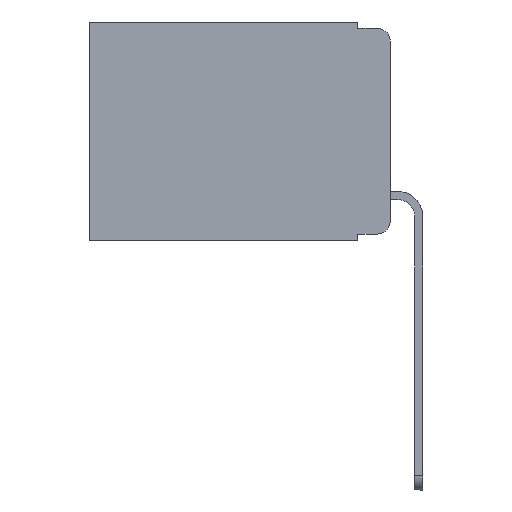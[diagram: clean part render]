
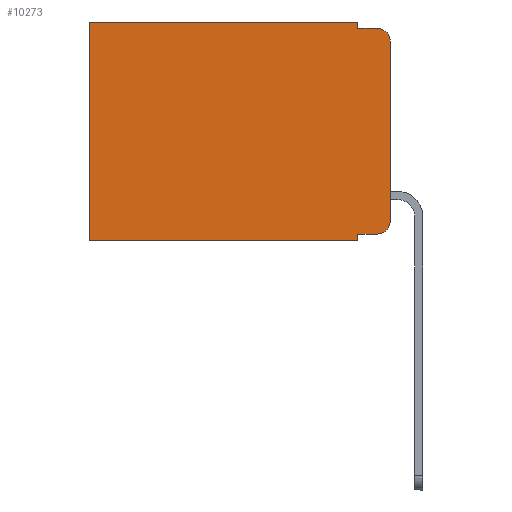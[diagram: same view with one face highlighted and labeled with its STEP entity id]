
A CAD part, left-side view. The second image highlights one B-rep face of the part: STEP entity #10273.
In plain terms, the highlighted planar face has unit normal (-1, 0, 0).
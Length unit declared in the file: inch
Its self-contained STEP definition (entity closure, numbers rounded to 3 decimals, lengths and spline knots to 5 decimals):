
#272 = FACE_OUTER_BOUND ( 'NONE', #5683, .T. ) ;
#402 = CARTESIAN_POINT ( 'NONE',  ( 0.298, 0.051, -0.333 ) ) ;
#705 = VERTEX_POINT ( 'NONE', #9964 ) ;
#1305 = VERTEX_POINT ( 'NONE', #12689 ) ;
#1468 = CIRCLE ( 'NONE', #20230, 0.02 ) ;
#1598 = ORIENTED_EDGE ( 'NONE', *, *, #20343, .F. ) ;
#1930 = PLANE ( 'NONE',  #18754 ) ;
#2007 = CARTESIAN_POINT ( 'NONE',  ( 0.298, 0.02, -0.03 ) ) ;
#2452 = CARTESIAN_POINT ( 'NONE',  ( 0.298, 0.02, -0.01 ) ) ;
#3586 = CARTESIAN_POINT ( 'NONE',  ( 0.298, 0., 0. ) ) ;
#3690 = LINE ( 'NONE', #3586, #3766 ) ;
#3766 = VECTOR ( 'NONE', #14109, 39.37008 ) ;
#3961 = VERTEX_POINT ( 'NONE', #14930 ) ;
#4015 = DIRECTION ( 'NONE',  ( 0., 0., -1. ) ) ;
#4137 = ORIENTED_EDGE ( 'NONE', *, *, #15783, .T. ) ;
#4173 = VECTOR ( 'NONE', #18829, 39.37008 ) ;
#4241 = CARTESIAN_POINT ( 'NONE',  ( 0.298, 0.473, 0. ) ) ;
#4502 = DIRECTION ( 'NONE',  ( -1., 0., 0. ) ) ;
#4708 = CARTESIAN_POINT ( 'NONE',  ( 0.298, 0.051, 0. ) ) ;
#5683 = EDGE_LOOP ( 'NONE', ( #20755, #4137, #12139, #21028, #20273, #18225, #15408, #1598, #11897, #7816 ) ) ;
#6067 = CARTESIAN_POINT ( 'NONE',  ( 0.298, 0., -0.313 ) ) ;
#6158 = VECTOR ( 'NONE', #13902, 39.37008 ) ;
#6461 = EDGE_CURVE ( 'NONE', #9004, #10953, #3690, .T. ) ;
#6889 = VECTOR ( 'NONE', #21784, 39.37008 ) ;
#7030 = DIRECTION ( 'NONE',  ( 1., 0., 0. ) ) ;
#7320 = CARTESIAN_POINT ( 'NONE',  ( 0.298, 0.473, 0. ) ) ;
#7493 = CARTESIAN_POINT ( 'NONE',  ( 0.298, 0.02, -0.313 ) ) ;
#7816 = ORIENTED_EDGE ( 'NONE', *, *, #12599, .T. ) ;
#8092 = LINE ( 'NONE', #9531, #14016 ) ;
#8158 = VERTEX_POINT ( 'NONE', #17077 ) ;
#8767 = DIRECTION ( 'NONE',  ( -1., 0., 0. ) ) ;
#8804 = CARTESIAN_POINT ( 'NONE',  ( 0.298, 0., 0. ) ) ;
#9004 = VERTEX_POINT ( 'NONE', #12047 ) ;
#9333 = VECTOR ( 'NONE', #21646, 39.37008 ) ;
#9531 = CARTESIAN_POINT ( 'NONE',  ( 0.298, 0.051, 0. ) ) ;
#9964 = CARTESIAN_POINT ( 'NONE',  ( 0.298, 0.051, -0.01 ) ) ;
#10273 = ADVANCED_FACE ( 'NONE', ( #272 ), #1930, .F. ) ;
#10521 = CARTESIAN_POINT ( 'NONE',  ( 0.298, 0.051, -0.01 ) ) ;
#10665 = CARTESIAN_POINT ( 'NONE',  ( 0.298, 0.051, -0.333 ) ) ;
#10953 = VERTEX_POINT ( 'NONE', #6067 ) ;
#11064 = VECTOR ( 'NONE', #4015, 39.37008 ) ;
#11520 = VECTOR ( 'NONE', #15269, 39.37008 ) ;
#11543 = LINE ( 'NONE', #13416, #9333 ) ;
#11897 = ORIENTED_EDGE ( 'NONE', *, *, #17903, .T. ) ;
#12047 = CARTESIAN_POINT ( 'NONE',  ( 0.298, 0., -0.03 ) ) ;
#12139 = ORIENTED_EDGE ( 'NONE', *, *, #21716, .F. ) ;
#12599 = EDGE_CURVE ( 'NONE', #8158, #10953, #1468, .T. ) ;
#12689 = CARTESIAN_POINT ( 'NONE',  ( 0.298, 0.051, 0. ) ) ;
#13270 = VERTEX_POINT ( 'NONE', #10665 ) ;
#13335 = LINE ( 'NONE', #4708, #6889 ) ;
#13416 = CARTESIAN_POINT ( 'NONE',  ( 0.298, 0., 0. ) ) ;
#13902 = DIRECTION ( 'NONE',  ( 0., -1., 0. ) ) ;
#14016 = VECTOR ( 'NONE', #14840, 39.37008 ) ;
#14109 = DIRECTION ( 'NONE',  ( 0., 0., -1. ) ) ;
#14168 = EDGE_CURVE ( 'NONE', #17175, #21309, #20979, .T. ) ;
#14840 = DIRECTION ( 'NONE',  ( 0., 0., -1. ) ) ;
#14930 = CARTESIAN_POINT ( 'NONE',  ( 0.298, 0.051, -0.343 ) ) ;
#15119 = CARTESIAN_POINT ( 'NONE',  ( 0.298, 0.473, -0.343 ) ) ;
#15269 = DIRECTION ( 'NONE',  ( 0., 1., 0. ) ) ;
#15350 = LINE ( 'NONE', #402, #6158 ) ;
#15408 = ORIENTED_EDGE ( 'NONE', *, *, #19172, .F. ) ;
#15783 = EDGE_CURVE ( 'NONE', #9004, #18899, #16078, .T. ) ;
#16078 = CIRCLE ( 'NONE', #17141, 0.02 ) ;
#16872 = EDGE_CURVE ( 'NONE', #1305, #17175, #11543, .T. ) ;
#16939 = LINE ( 'NONE', #18820, #11520 ) ;
#17077 = CARTESIAN_POINT ( 'NONE',  ( 0.298, 0.02, -0.333 ) ) ;
#17141 = AXIS2_PLACEMENT_3D ( 'NONE', #2007, #8767, #20730 ) ;
#17175 = VERTEX_POINT ( 'NONE', #7320 ) ;
#17903 = EDGE_CURVE ( 'NONE', #13270, #8158, #15350, .T. ) ;
#17908 = DIRECTION ( 'NONE',  ( 0., 0., -1. ) ) ;
#18174 = EDGE_CURVE ( 'NONE', #1305, #705, #13335, .T. ) ;
#18225 = ORIENTED_EDGE ( 'NONE', *, *, #14168, .T. ) ;
#18754 = AXIS2_PLACEMENT_3D ( 'NONE', #8804, #7030, #18882 ) ;
#18820 = CARTESIAN_POINT ( 'NONE',  ( 0.298, 0., -0.343 ) ) ;
#18829 = DIRECTION ( 'NONE',  ( 0., -1., 0. ) ) ;
#18882 = DIRECTION ( 'NONE',  ( 0., 0., -1. ) ) ;
#18899 = VERTEX_POINT ( 'NONE', #2452 ) ;
#19172 = EDGE_CURVE ( 'NONE', #3961, #21309, #16939, .T. ) ;
#20230 = AXIS2_PLACEMENT_3D ( 'NONE', #7493, #4502, #17908 ) ;
#20273 = ORIENTED_EDGE ( 'NONE', *, *, #16872, .T. ) ;
#20285 = LINE ( 'NONE', #10521, #4173 ) ;
#20343 = EDGE_CURVE ( 'NONE', #13270, #3961, #8092, .T. ) ;
#20730 = DIRECTION ( 'NONE',  ( 0., 0., -1. ) ) ;
#20755 = ORIENTED_EDGE ( 'NONE', *, *, #6461, .F. ) ;
#20979 = LINE ( 'NONE', #4241, #11064 ) ;
#21028 = ORIENTED_EDGE ( 'NONE', *, *, #18174, .F. ) ;
#21309 = VERTEX_POINT ( 'NONE', #15119 ) ;
#21646 = DIRECTION ( 'NONE',  ( 0., 1., 0. ) ) ;
#21716 = EDGE_CURVE ( 'NONE', #705, #18899, #20285, .T. ) ;
#21784 = DIRECTION ( 'NONE',  ( 0., 0., -1. ) ) ;
